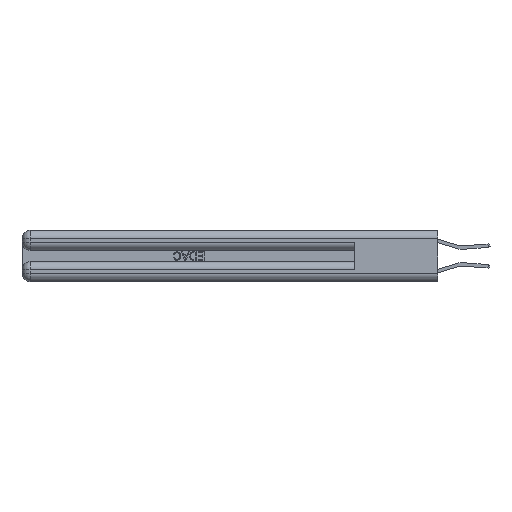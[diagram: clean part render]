
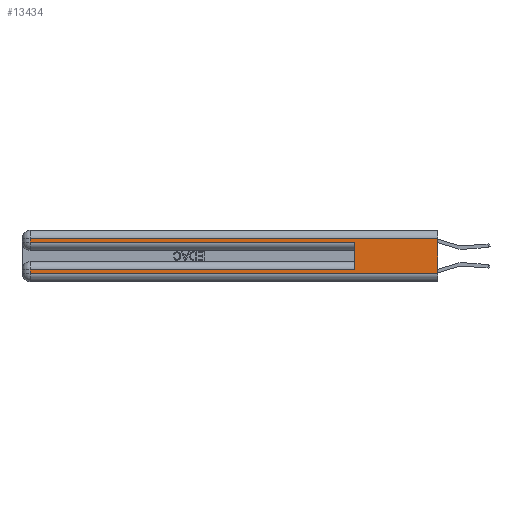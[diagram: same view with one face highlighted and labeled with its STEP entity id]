
A CAD part, left-side view. The second image highlights one B-rep face of the part: STEP entity #13434.
In plain terms, the highlighted planar face has unit normal (-1, 0, 0).
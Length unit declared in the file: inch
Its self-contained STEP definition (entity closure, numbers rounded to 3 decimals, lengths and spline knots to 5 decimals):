
#134 = CARTESIAN_POINT ( 'NONE',  ( 0., 0., 0.37 ) ) ;
#562 = EDGE_CURVE ( 'NONE', #7796, #28547, #31249, .T. ) ;
#886 = EDGE_CURVE ( 'NONE', #29999, #33077, #19167, .T. ) ;
#1908 = VECTOR ( 'NONE', #16312, 39.37008 ) ;
#2153 = CARTESIAN_POINT ( 'NONE',  ( 0., 0., 0.085 ) ) ;
#2214 = LINE ( 'NONE', #29212, #32990 ) ;
#2927 = VERTEX_POINT ( 'NONE', #32194 ) ;
#3586 = ORIENTED_EDGE ( 'NONE', *, *, #4565, .T. ) ;
#4565 = EDGE_CURVE ( 'NONE', #33077, #31651, #31091, .T. ) ;
#5015 = DIRECTION ( 'NONE',  ( 0., 0., -1. ) ) ;
#5108 = VECTOR ( 'NONE', #5015, 39.37008 ) ;
#5192 = VECTOR ( 'NONE', #28564, 39.37008 ) ;
#5807 = CARTESIAN_POINT ( 'NONE',  ( 0., 0., 0.06 ) ) ;
#7091 = EDGE_CURVE ( 'NONE', #19713, #2927, #10228, .T. ) ;
#7144 = AXIS2_PLACEMENT_3D ( 'NONE', #21066, #9635, #9457 ) ;
#7796 = VERTEX_POINT ( 'NONE', #22666 ) ;
#9272 = FACE_OUTER_BOUND ( 'NONE', #24004, .T. ) ;
#9457 = DIRECTION ( 'NONE',  ( 0., 0., -1. ) ) ;
#9547 = EDGE_CURVE ( 'NONE', #31465, #19713, #27499, .T. ) ;
#9635 = DIRECTION ( 'NONE',  ( 1., 0., 0. ) ) ;
#10228 = LINE ( 'NONE', #21292, #22741 ) ;
#10467 = CARTESIAN_POINT ( 'NONE',  ( 0., 0.6, 0.285 ) ) ;
#10550 = DIRECTION ( 'NONE',  ( 0., 0., 1. ) ) ;
#11394 = CARTESIAN_POINT ( 'NONE',  ( 0., 0., 0.285 ) ) ;
#11737 = CARTESIAN_POINT ( 'NONE',  ( 0., 2.94, 0.285 ) ) ;
#11788 = VECTOR ( 'NONE', #33448, 39.37008 ) ;
#12175 = PLANE ( 'NONE',  #7144 ) ;
#12197 = CARTESIAN_POINT ( 'NONE',  ( 0., 2.94, 0.085 ) ) ;
#12514 = CARTESIAN_POINT ( 'NONE',  ( 0., 0., 0.31 ) ) ;
#13434 = ADVANCED_FACE ( 'NONE', ( #9272 ), #12175, .F. ) ;
#15397 = ORIENTED_EDGE ( 'NONE', *, *, #562, .F. ) ;
#15967 = CARTESIAN_POINT ( 'NONE',  ( 0., 2.94, 0.31 ) ) ;
#16312 = DIRECTION ( 'NONE',  ( 0., 1., 0. ) ) ;
#16755 = EDGE_CURVE ( 'NONE', #31465, #31651, #2214, .T. ) ;
#19167 = LINE ( 'NONE', #29973, #5108 ) ;
#19405 = VECTOR ( 'NONE', #25727, 39.37008 ) ;
#19713 = VERTEX_POINT ( 'NONE', #12197 ) ;
#19820 = VECTOR ( 'NONE', #27901, 39.37008 ) ;
#20082 = EDGE_CURVE ( 'NONE', #2927, #28547, #30430, .T. ) ;
#21066 = CARTESIAN_POINT ( 'NONE',  ( 0., 0., 0.37 ) ) ;
#21177 = ORIENTED_EDGE ( 'NONE', *, *, #16755, .F. ) ;
#21292 = CARTESIAN_POINT ( 'NONE',  ( 0., 2.94, 0.37 ) ) ;
#22666 = CARTESIAN_POINT ( 'NONE',  ( 0., 0., 0.31 ) ) ;
#22741 = VECTOR ( 'NONE', #32285, 39.37008 ) ;
#24004 = EDGE_LOOP ( 'NONE', ( #15397, #33995, #35225, #3586, #21177, #35027, #26010, #32829 ) ) ;
#25727 = DIRECTION ( 'NONE',  ( 0., 1., 0. ) ) ;
#26010 = ORIENTED_EDGE ( 'NONE', *, *, #7091, .T. ) ;
#27499 = LINE ( 'NONE', #2153, #1908 ) ;
#27901 = DIRECTION ( 'NONE',  ( 0., -1., 0. ) ) ;
#28547 = VERTEX_POINT ( 'NONE', #31497 ) ;
#28564 = DIRECTION ( 'NONE',  ( 0., 0., -1. ) ) ;
#28793 = LINE ( 'NONE', #12514, #19405 ) ;
#29212 = CARTESIAN_POINT ( 'NONE',  ( 0., 0.6, 0.145 ) ) ;
#29973 = CARTESIAN_POINT ( 'NONE',  ( 0., 2.94, 0.37 ) ) ;
#29999 = VERTEX_POINT ( 'NONE', #15967 ) ;
#30430 = LINE ( 'NONE', #5807, #19820 ) ;
#31091 = LINE ( 'NONE', #11394, #11788 ) ;
#31249 = LINE ( 'NONE', #134, #5192 ) ;
#31465 = VERTEX_POINT ( 'NONE', #32176 ) ;
#31497 = CARTESIAN_POINT ( 'NONE',  ( 0., 0., 0.06 ) ) ;
#31651 = VERTEX_POINT ( 'NONE', #10467 ) ;
#32176 = CARTESIAN_POINT ( 'NONE',  ( 0., 0.6, 0.085 ) ) ;
#32194 = CARTESIAN_POINT ( 'NONE',  ( 0., 2.94, 0.06 ) ) ;
#32285 = DIRECTION ( 'NONE',  ( 0., 0., -1. ) ) ;
#32829 = ORIENTED_EDGE ( 'NONE', *, *, #20082, .T. ) ;
#32990 = VECTOR ( 'NONE', #10550, 39.37008 ) ;
#33077 = VERTEX_POINT ( 'NONE', #11737 ) ;
#33448 = DIRECTION ( 'NONE',  ( 0., -1., 0. ) ) ;
#33995 = ORIENTED_EDGE ( 'NONE', *, *, #35497, .T. ) ;
#35027 = ORIENTED_EDGE ( 'NONE', *, *, #9547, .T. ) ;
#35225 = ORIENTED_EDGE ( 'NONE', *, *, #886, .T. ) ;
#35497 = EDGE_CURVE ( 'NONE', #7796, #29999, #28793, .T. ) ;
